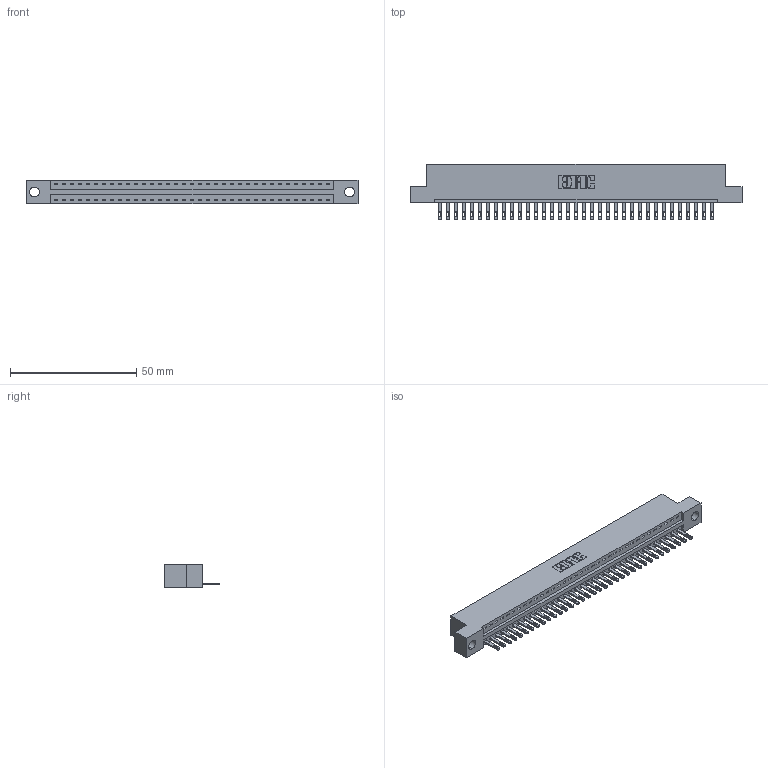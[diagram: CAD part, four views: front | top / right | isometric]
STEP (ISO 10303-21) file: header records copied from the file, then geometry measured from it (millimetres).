
FILE_DESCRIPTION (( 'STEP AP203' ), '1' );
FILE_NAME ('346-035-500-104.STEP', '2018-08-23T23:37:54', ( '' ), ( '' ), 'SwSTEP 2.0', 'SolidWorks 2016', '' );
FILE_SCHEMA (( 'CONFIG_CONTROL_DESIGN' ));
Length unit declared in the file: inch
Products named in the file (3): 346 Part_Flush Mounting Lugs - 0.156 Dia-TH; 345-292-001_345-293-100; 346-035-500-104
Assembly tree (36 placements, depth 2):
  346-035-500-104
    346 Part_Flush Mounting Lugs - 0.156 Dia-TH
    345-292-001_345-293-100  x35
Bounding box: 131.7 x 21.84 x 9.4 mm (x, y, z)
Volume: 12492.1 mm3; surface area: 15424.5 mm2
Topology: 36 solids, 36 shells, 2012 faces, 6209 edges, 4138 vertices
Faces by surface type: plane 1266, cylinder 746
Entity records: 22597 total; most frequent: CARTESIAN_POINT 3881, ORIENTED_EDGE 3850, DIRECTION 3435, EDGE_CURVE 1925, LINE 1649, VECTOR 1649, VERTEX_POINT 1282, AXIS2_PLACEMENT_3D 893
